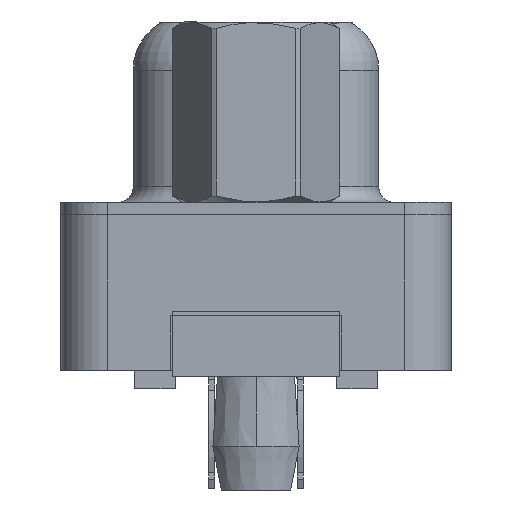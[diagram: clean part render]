
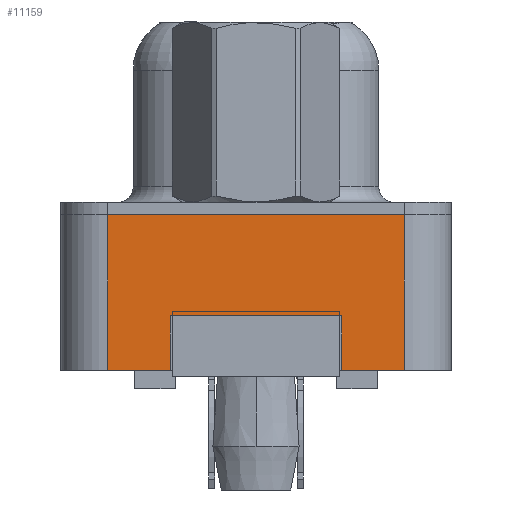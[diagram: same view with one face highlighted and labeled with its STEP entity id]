
A CAD part, left-side view. The second image highlights one B-rep face of the part: STEP entity #11159.
In plain terms, the highlighted planar face has unit normal (-1, 0, 0).
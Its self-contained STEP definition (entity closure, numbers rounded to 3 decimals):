
#659 = CARTESIAN_POINT ( 'NONE',  ( -2.91, -4.775, -5. ) ) ;
#1056 = CARTESIAN_POINT ( 'NONE',  ( -2.91, 2.75, -5. ) ) ;
#1497 = CARTESIAN_POINT ( 'NONE',  ( -2.91, 2.75, -3.25 ) ) ;
#1834 = ORIENTED_EDGE ( 'NONE', *, *, #6002, .F. ) ;
#2167 = EDGE_CURVE ( 'NONE', #6819, #13953, #16889, .T. ) ;
#2575 = VECTOR ( 'NONE', #3971, 1000. ) ;
#3971 = DIRECTION ( 'NONE',  ( 0., 0., -1. ) ) ;
#4224 = ORIENTED_EDGE ( 'NONE', *, *, #20712, .T. ) ;
#4770 = VECTOR ( 'NONE', #14483, 1000. ) ;
#5063 = LINE ( 'NONE', #18582, #21213 ) ;
#5153 = CARTESIAN_POINT ( 'NONE',  ( -2.91, -4.775, -5. ) ) ;
#5373 = ORIENTED_EDGE ( 'NONE', *, *, #16248, .F. ) ;
#5766 = VECTOR ( 'NONE', #5776, 1000. ) ;
#5776 = DIRECTION ( 'NONE',  ( 0., -1., 0. ) ) ;
#5956 = DIRECTION ( 'NONE',  ( 0., 1., 0. ) ) ;
#6002 = EDGE_CURVE ( 'NONE', #6819, #8425, #5063, .T. ) ;
#6137 = CARTESIAN_POINT ( 'NONE',  ( -2.91, -4.775, -5. ) ) ;
#6819 = VERTEX_POINT ( 'NONE', #22546 ) ;
#8155 = ORIENTED_EDGE ( 'NONE', *, *, #17925, .F. ) ;
#8425 = VERTEX_POINT ( 'NONE', #9457 ) ;
#9457 = CARTESIAN_POINT ( 'NONE',  ( -2.91, 4.775, 0. ) ) ;
#10020 = CARTESIAN_POINT ( 'NONE',  ( -2.91, 2.75, -3.25 ) ) ;
#10205 = ORIENTED_EDGE ( 'NONE', *, *, #13035, .F. ) ;
#10593 = LINE ( 'NONE', #26547, #17686 ) ;
#10597 = VECTOR ( 'NONE', #12886, 1000. ) ;
#11159 = ADVANCED_FACE ( 'NONE', ( #15297 ), #24047, .T. ) ;
#11198 = VERTEX_POINT ( 'NONE', #24481 ) ;
#11415 = ORIENTED_EDGE ( 'NONE', *, *, #12738, .T. ) ;
#12738 = EDGE_CURVE ( 'NONE', #23027, #11198, #24562, .T. ) ;
#12886 = DIRECTION ( 'NONE',  ( 0., 0., 1. ) ) ;
#13035 = EDGE_CURVE ( 'NONE', #23367, #13953, #19044, .T. ) ;
#13537 = EDGE_LOOP ( 'NONE', ( #11415, #18525, #4224, #5373, #1834, #14749, #10205, #8155 ) ) ;
#13783 = VECTOR ( 'NONE', #18559, 1000. ) ;
#13953 = VERTEX_POINT ( 'NONE', #1056 ) ;
#14483 = DIRECTION ( 'NONE',  ( 0., -1., 0. ) ) ;
#14749 = ORIENTED_EDGE ( 'NONE', *, *, #2167, .T. ) ;
#15155 = CARTESIAN_POINT ( 'NONE',  ( -2.91, -4.775, -5. ) ) ;
#15229 = CARTESIAN_POINT ( 'NONE',  ( -2.91, -2.75, -3.25 ) ) ;
#15297 = FACE_OUTER_BOUND ( 'NONE', #13537, .T. ) ;
#16003 = AXIS2_PLACEMENT_3D ( 'NONE', #15155, #19833, #26462 ) ;
#16248 = EDGE_CURVE ( 'NONE', #8425, #29211, #21291, .T. ) ;
#16782 = DIRECTION ( 'NONE',  ( 0., 0., 1. ) ) ;
#16889 = LINE ( 'NONE', #5153, #4770 ) ;
#17686 = VECTOR ( 'NONE', #5956, 1000. ) ;
#17925 = EDGE_CURVE ( 'NONE', #23027, #23367, #10593, .T. ) ;
#18271 = CARTESIAN_POINT ( 'NONE',  ( -2.91, -4.775, 0. ) ) ;
#18525 = ORIENTED_EDGE ( 'NONE', *, *, #18973, .T. ) ;
#18559 = DIRECTION ( 'NONE',  ( 0., -1., 0. ) ) ;
#18582 = CARTESIAN_POINT ( 'NONE',  ( -2.91, 4.775, -5. ) ) ;
#18973 = EDGE_CURVE ( 'NONE', #11198, #23935, #24255, .T. ) ;
#19044 = LINE ( 'NONE', #10020, #26588 ) ;
#19265 = CARTESIAN_POINT ( 'NONE',  ( -2.91, -2.75, -3.25 ) ) ;
#19833 = DIRECTION ( 'NONE',  ( -1., 0., 0. ) ) ;
#20712 = EDGE_CURVE ( 'NONE', #23935, #29211, #26592, .T. ) ;
#21213 = VECTOR ( 'NONE', #16782, 1000. ) ;
#21291 = LINE ( 'NONE', #18271, #13783 ) ;
#21548 = CARTESIAN_POINT ( 'NONE',  ( -2.91, -4.775, -5. ) ) ;
#22546 = CARTESIAN_POINT ( 'NONE',  ( -2.91, 4.775, -5. ) ) ;
#23027 = VERTEX_POINT ( 'NONE', #19265 ) ;
#23092 = CARTESIAN_POINT ( 'NONE',  ( -2.91, -4.775, 0. ) ) ;
#23367 = VERTEX_POINT ( 'NONE', #1497 ) ;
#23935 = VERTEX_POINT ( 'NONE', #659 ) ;
#24047 = PLANE ( 'NONE',  #16003 ) ;
#24255 = LINE ( 'NONE', #21548, #5766 ) ;
#24481 = CARTESIAN_POINT ( 'NONE',  ( -2.91, -2.75, -5. ) ) ;
#24562 = LINE ( 'NONE', #15229, #2575 ) ;
#26127 = DIRECTION ( 'NONE',  ( 0., 0., -1. ) ) ;
#26462 = DIRECTION ( 'NONE',  ( 0., 0., 1. ) ) ;
#26547 = CARTESIAN_POINT ( 'NONE',  ( -2.91, 2.75, -3.25 ) ) ;
#26588 = VECTOR ( 'NONE', #26127, 1000. ) ;
#26592 = LINE ( 'NONE', #6137, #10597 ) ;
#29211 = VERTEX_POINT ( 'NONE', #23092 ) ;
